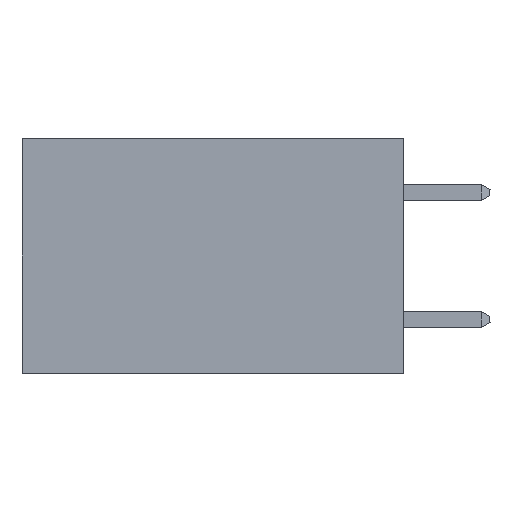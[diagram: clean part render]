
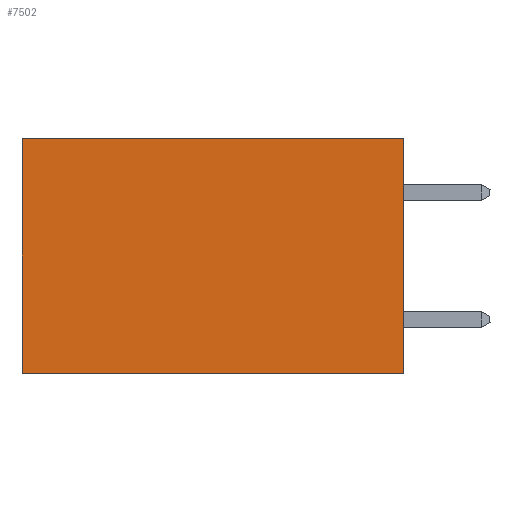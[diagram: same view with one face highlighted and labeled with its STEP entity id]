
A CAD part, left-side view. The second image highlights one B-rep face of the part: STEP entity #7502.
In plain terms, the highlighted planar face has unit normal (-1, 0, 0).
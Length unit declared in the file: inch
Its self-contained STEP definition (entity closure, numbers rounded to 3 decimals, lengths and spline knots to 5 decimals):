
#907 = EDGE_CURVE ( 'NONE', #11884, #3113, #2121, .T. ) ;
#1176 = DIRECTION ( 'NONE',  ( 0., 0., -1. ) ) ;
#1514 = LINE ( 'NONE', #4416, #3409 ) ;
#2098 = CARTESIAN_POINT ( 'NONE',  ( 0.2875, 0., -0.37 ) ) ;
#2121 = LINE ( 'NONE', #12515, #10380 ) ;
#2888 = CARTESIAN_POINT ( 'NONE',  ( 0.2875, 0.6, 0. ) ) ;
#3113 = VERTEX_POINT ( 'NONE', #6482 ) ;
#3347 = ORIENTED_EDGE ( 'NONE', *, *, #3939, .F. ) ;
#3409 = VECTOR ( 'NONE', #7453, 39.37008 ) ;
#3904 = EDGE_CURVE ( 'NONE', #4638, #6686, #1514, .T. ) ;
#3939 = EDGE_CURVE ( 'NONE', #4638, #11884, #5994, .T. ) ;
#4154 = PLANE ( 'NONE',  #6892 ) ;
#4416 = CARTESIAN_POINT ( 'NONE',  ( 0.2875, 0., 0. ) ) ;
#4638 = VERTEX_POINT ( 'NONE', #7241 ) ;
#4846 = LINE ( 'NONE', #2888, #5473 ) ;
#5473 = VECTOR ( 'NONE', #10144, 39.37008 ) ;
#5833 = EDGE_LOOP ( 'NONE', ( #6387, #7915, #3347, #6068 ) ) ;
#5994 = LINE ( 'NONE', #11472, #10723 ) ;
#6068 = ORIENTED_EDGE ( 'NONE', *, *, #3904, .T. ) ;
#6387 = ORIENTED_EDGE ( 'NONE', *, *, #10521, .T. ) ;
#6482 = CARTESIAN_POINT ( 'NONE',  ( 0.2875, 0.6, -0.37 ) ) ;
#6686 = VERTEX_POINT ( 'NONE', #11939 ) ;
#6892 = AXIS2_PLACEMENT_3D ( 'NONE', #12323, #7284, #1176 ) ;
#7241 = CARTESIAN_POINT ( 'NONE',  ( 0.2875, 0., 0. ) ) ;
#7284 = DIRECTION ( 'NONE',  ( 1., 0., 0. ) ) ;
#7453 = DIRECTION ( 'NONE',  ( 0., 1., 0. ) ) ;
#7502 = ADVANCED_FACE ( 'NONE', ( #12715 ), #4154, .F. ) ;
#7915 = ORIENTED_EDGE ( 'NONE', *, *, #907, .F. ) ;
#9508 = DIRECTION ( 'NONE',  ( 0., 0., -1. ) ) ;
#10144 = DIRECTION ( 'NONE',  ( 0., 0., -1. ) ) ;
#10380 = VECTOR ( 'NONE', #12697, 39.37008 ) ;
#10521 = EDGE_CURVE ( 'NONE', #6686, #3113, #4846, .T. ) ;
#10723 = VECTOR ( 'NONE', #9508, 39.37008 ) ;
#11472 = CARTESIAN_POINT ( 'NONE',  ( 0.2875, 0., 0. ) ) ;
#11884 = VERTEX_POINT ( 'NONE', #2098 ) ;
#11939 = CARTESIAN_POINT ( 'NONE',  ( 0.2875, 0.6, 0. ) ) ;
#12323 = CARTESIAN_POINT ( 'NONE',  ( 0.2875, 0., 0. ) ) ;
#12515 = CARTESIAN_POINT ( 'NONE',  ( 0.2875, 0., -0.37 ) ) ;
#12697 = DIRECTION ( 'NONE',  ( 0., 1., 0. ) ) ;
#12715 = FACE_OUTER_BOUND ( 'NONE', #5833, .T. ) ;
